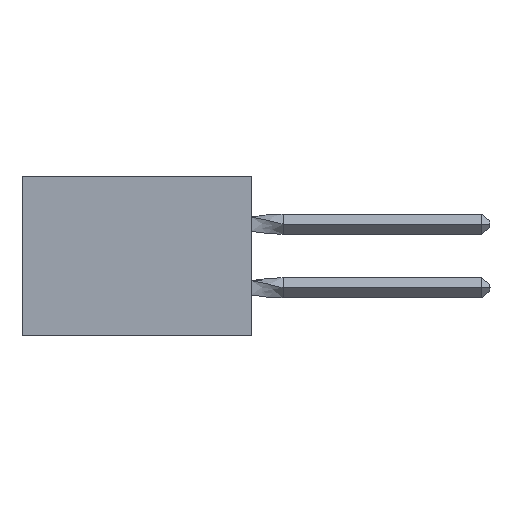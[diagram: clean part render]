
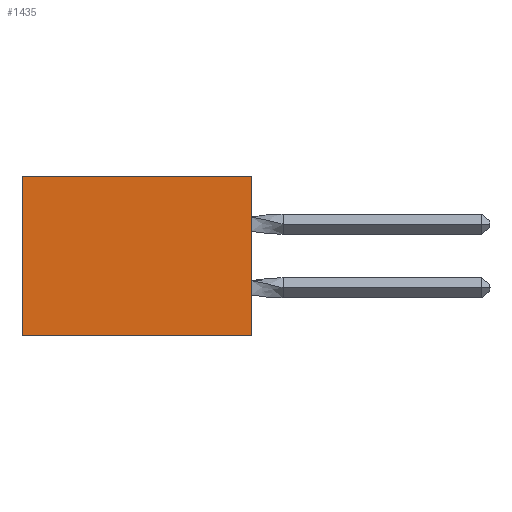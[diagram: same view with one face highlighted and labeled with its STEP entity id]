
A CAD part, left-side view. The second image highlights one B-rep face of the part: STEP entity #1435.
In plain terms, the highlighted planar face has unit normal (-1, 0, 0).
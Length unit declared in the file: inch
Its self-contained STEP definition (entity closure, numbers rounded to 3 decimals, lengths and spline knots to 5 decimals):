
#1435 = ADVANCED_FACE ( 'NONE', ( #4395 ), #11902, .F. ) ;
#1543 = VECTOR ( 'NONE', #2360, 39.37008 ) ;
#2360 = DIRECTION ( 'NONE',  ( 0., 0., -1. ) ) ;
#2502 = AXIS2_PLACEMENT_3D ( 'NONE', #5225, #7640, #5266 ) ;
#2685 = VERTEX_POINT ( 'NONE', #13810 ) ;
#2753 = LINE ( 'NONE', #11895, #8389 ) ;
#2881 = VERTEX_POINT ( 'NONE', #10815 ) ;
#4308 = ORIENTED_EDGE ( 'NONE', *, *, #5749, .T. ) ;
#4395 = FACE_OUTER_BOUND ( 'NONE', #14308, .T. ) ;
#4804 = DIRECTION ( 'NONE',  ( 0., 1., 0. ) ) ;
#4947 = LINE ( 'NONE', #6028, #10714 ) ;
#5225 = CARTESIAN_POINT ( 'NONE',  ( 0.305, 0., -0.5 ) ) ;
#5266 = DIRECTION ( 'NONE',  ( 0., 0., -1. ) ) ;
#5507 = EDGE_CURVE ( 'NONE', #6884, #8484, #9608, .T. ) ;
#5749 = EDGE_CURVE ( 'NONE', #6884, #2881, #2753, .T. ) ;
#5838 = ORIENTED_EDGE ( 'NONE', *, *, #13510, .F. ) ;
#5923 = DIRECTION ( 'NONE',  ( 0., 0., -1. ) ) ;
#5948 = ORIENTED_EDGE ( 'NONE', *, *, #5507, .F. ) ;
#6028 = CARTESIAN_POINT ( 'NONE',  ( 0.305, 0., -0.5 ) ) ;
#6268 = CARTESIAN_POINT ( 'NONE',  ( 0.305, 0., 0. ) ) ;
#6532 = CARTESIAN_POINT ( 'NONE',  ( 0.305, 0., -0.5 ) ) ;
#6884 = VERTEX_POINT ( 'NONE', #6268 ) ;
#7640 = DIRECTION ( 'NONE',  ( 1., 0., 0. ) ) ;
#8389 = VECTOR ( 'NONE', #11950, 39.37008 ) ;
#8484 = VERTEX_POINT ( 'NONE', #6532 ) ;
#9191 = EDGE_CURVE ( 'NONE', #2881, #2685, #10360, .T. ) ;
#9608 = LINE ( 'NONE', #11326, #1543 ) ;
#10360 = LINE ( 'NONE', #11287, #11561 ) ;
#10714 = VECTOR ( 'NONE', #4804, 39.37008 ) ;
#10815 = CARTESIAN_POINT ( 'NONE',  ( 0.305, 0.72, 0. ) ) ;
#11287 = CARTESIAN_POINT ( 'NONE',  ( 0.305, 0.72, -0.5 ) ) ;
#11326 = CARTESIAN_POINT ( 'NONE',  ( 0.305, 0., -0.5 ) ) ;
#11561 = VECTOR ( 'NONE', #5923, 39.37008 ) ;
#11895 = CARTESIAN_POINT ( 'NONE',  ( 0.305, 0., 0. ) ) ;
#11902 = PLANE ( 'NONE',  #2502 ) ;
#11950 = DIRECTION ( 'NONE',  ( 0., 1., 0. ) ) ;
#13510 = EDGE_CURVE ( 'NONE', #8484, #2685, #4947, .T. ) ;
#13810 = CARTESIAN_POINT ( 'NONE',  ( 0.305, 0.72, -0.5 ) ) ;
#14029 = ORIENTED_EDGE ( 'NONE', *, *, #9191, .T. ) ;
#14308 = EDGE_LOOP ( 'NONE', ( #14029, #5838, #5948, #4308 ) ) ;
